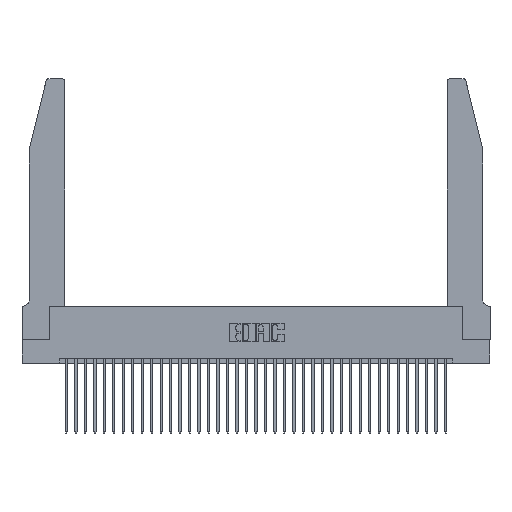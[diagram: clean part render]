
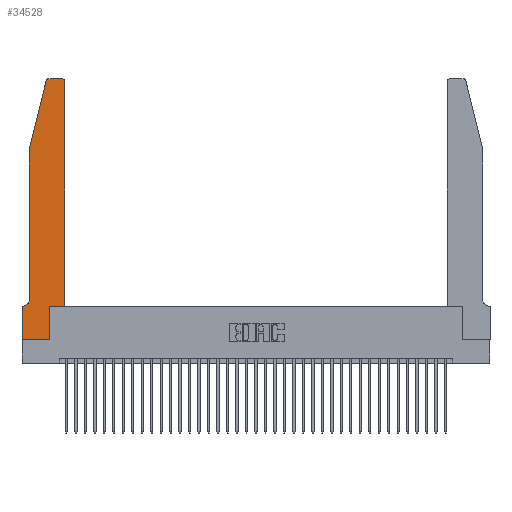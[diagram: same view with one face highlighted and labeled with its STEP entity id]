
A CAD part, top view. The second image highlights one B-rep face of the part: STEP entity #34528.
In plain terms, the highlighted planar face has unit normal (0, 0, 1).
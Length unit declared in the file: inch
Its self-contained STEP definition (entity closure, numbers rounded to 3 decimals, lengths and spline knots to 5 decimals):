
#1128 = VERTEX_POINT ( 'NONE', #4795 ) ;
#1142 = LINE ( 'NONE', #27657, #16571 ) ;
#1581 = CIRCLE ( 'NONE', #6275, 0.03 ) ;
#1779 = VERTEX_POINT ( 'NONE', #21630 ) ;
#1980 = DIRECTION ( 'NONE',  ( 0., 0., 1. ) ) ;
#2965 = EDGE_CURVE ( 'NONE', #1128, #6114, #33499, .T. ) ;
#3066 = DIRECTION ( 'NONE',  ( 0., 1., 0. ) ) ;
#3190 = VECTOR ( 'NONE', #3066, 39.37008 ) ;
#3422 = ORIENTED_EDGE ( 'NONE', *, *, #18337, .T. ) ;
#3525 = VECTOR ( 'NONE', #30238, 39.37008 ) ;
#4795 = CARTESIAN_POINT ( 'NONE',  ( 0., 0., 0.37 ) ) ;
#4916 = CARTESIAN_POINT ( 'NONE',  ( 0., 0.35, 0.37 ) ) ;
#5437 = EDGE_CURVE ( 'NONE', #25850, #1779, #28876, .T. ) ;
#5640 = VERTEX_POINT ( 'NONE', #32951 ) ;
#5647 = ORIENTED_EDGE ( 'NONE', *, *, #13364, .T. ) ;
#5784 = LINE ( 'NONE', #11953, #35310 ) ;
#6114 = VERTEX_POINT ( 'NONE', #34794 ) ;
#6275 = AXIS2_PLACEMENT_3D ( 'NONE', #12377, #32295, #15337 ) ;
#6824 = VERTEX_POINT ( 'NONE', #9285 ) ;
#8579 = CARTESIAN_POINT ( 'NONE',  ( 0.0755, 0.35, 0.37 ) ) ;
#8864 = ORIENTED_EDGE ( 'NONE', *, *, #36455, .T. ) ;
#9285 = CARTESIAN_POINT ( 'NONE',  ( 0.2865, 0.35, 0.37 ) ) ;
#10148 = EDGE_CURVE ( 'NONE', #16829, #36182, #36560, .T. ) ;
#10251 = VERTEX_POINT ( 'NONE', #15287 ) ;
#10747 = PLANE ( 'NONE',  #29472 ) ;
#11078 = CARTESIAN_POINT ( 'NONE',  ( 0.0755, 2., 0.37 ) ) ;
#11239 = LINE ( 'NONE', #24502, #3525 ) ;
#11369 = VECTOR ( 'NONE', #16510, 39.37008 ) ;
#11953 = CARTESIAN_POINT ( 'NONE',  ( 0.4505, 0.35, 0.37 ) ) ;
#12377 = CARTESIAN_POINT ( 'NONE',  ( 0.4205, 2.72, 0.37 ) ) ;
#13364 = EDGE_CURVE ( 'NONE', #36182, #27107, #31470, .T. ) ;
#13442 = CARTESIAN_POINT ( 'NONE',  ( 0.0055, 0.42, 0.37 ) ) ;
#13700 = DIRECTION ( 'NONE',  ( 0., 0., 1. ) ) ;
#14864 = DIRECTION ( 'NONE',  ( 0., -1., 0. ) ) ;
#15026 = DIRECTION ( 'NONE',  ( 1., 0., 0. ) ) ;
#15252 = ORIENTED_EDGE ( 'NONE', *, *, #5437, .T. ) ;
#15287 = CARTESIAN_POINT ( 'NONE',  ( 0.0055, 0.35, 0.37 ) ) ;
#15337 = DIRECTION ( 'NONE',  ( 1., 0., 0. ) ) ;
#16132 = AXIS2_PLACEMENT_3D ( 'NONE', #19301, #1980, #22150 ) ;
#16160 = VECTOR ( 'NONE', #20067, 39.37008 ) ;
#16347 = DIRECTION ( 'NONE',  ( -1., 0., 0. ) ) ;
#16509 = EDGE_CURVE ( 'NONE', #1779, #10251, #27436, .T. ) ;
#16510 = DIRECTION ( 'NONE',  ( -0.239, -0.971, 0. ) ) ;
#16571 = VECTOR ( 'NONE', #33372, 39.37008 ) ;
#16829 = VERTEX_POINT ( 'NONE', #23500 ) ;
#17015 = ORIENTED_EDGE ( 'NONE', *, *, #36226, .T. ) ;
#17113 = FACE_OUTER_BOUND ( 'NONE', #20928, .T. ) ;
#18337 = EDGE_CURVE ( 'NONE', #5640, #1128, #11239, .T. ) ;
#18440 = VECTOR ( 'NONE', #23781, 39.37008 ) ;
#19230 = CARTESIAN_POINT ( 'NONE',  ( 0.0755, 2., 0.37 ) ) ;
#19301 = CARTESIAN_POINT ( 'NONE',  ( 0.284, 2.72, 0.37 ) ) ;
#20067 = DIRECTION ( 'NONE',  ( -1., 0., 0. ) ) ;
#20123 = ORIENTED_EDGE ( 'NONE', *, *, #10148, .T. ) ;
#20928 = EDGE_LOOP ( 'NONE', ( #20123, #5647, #29405, #15252, #30307, #17015, #3422, #33862, #21457, #36520, #8864, #25871 ) ) ;
#21457 = ORIENTED_EDGE ( 'NONE', *, *, #29606, .T. ) ;
#21630 = CARTESIAN_POINT ( 'NONE',  ( 0.0755, 0.42, 0.37 ) ) ;
#22150 = DIRECTION ( 'NONE',  ( 1., 0., 0. ) ) ;
#22224 = VECTOR ( 'NONE', #14864, 39.37008 ) ;
#22645 = CARTESIAN_POINT ( 'NONE',  ( 0.284, 2.75, 0.37 ) ) ;
#23500 = CARTESIAN_POINT ( 'NONE',  ( 0.4205, 2.75, 0.37 ) ) ;
#23781 = DIRECTION ( 'NONE',  ( 1., 0., 0. ) ) ;
#24502 = CARTESIAN_POINT ( 'NONE',  ( 0., 0., 0.37 ) ) ;
#25086 = CARTESIAN_POINT ( 'NONE',  ( 0.4505, 0.35, 0.37 ) ) ;
#25850 = VERTEX_POINT ( 'NONE', #11078 ) ;
#25871 = ORIENTED_EDGE ( 'NONE', *, *, #26482, .T. ) ;
#26066 = CARTESIAN_POINT ( 'NONE',  ( 0.4505, 2.72, 0.37 ) ) ;
#26072 = LINE ( 'NONE', #34483, #3190 ) ;
#26475 = AXIS2_PLACEMENT_3D ( 'NONE', #13442, #33327, #16347 ) ;
#26482 = EDGE_CURVE ( 'NONE', #28957, #16829, #1581, .T. ) ;
#26630 = CARTESIAN_POINT ( 'NONE',  ( 0., 0., 0.37 ) ) ;
#27107 = VERTEX_POINT ( 'NONE', #35474 ) ;
#27436 = CIRCLE ( 'NONE', #26475, 0.07 ) ;
#27657 = CARTESIAN_POINT ( 'NONE',  ( 0.4505, 0.35, 0.37 ) ) ;
#28876 = LINE ( 'NONE', #31840, #22224 ) ;
#28957 = VERTEX_POINT ( 'NONE', #26066 ) ;
#29021 = VECTOR ( 'NONE', #34614, 39.37008 ) ;
#29221 = LINE ( 'NONE', #19230, #11369 ) ;
#29354 = EDGE_CURVE ( 'NONE', #27107, #25850, #29221, .T. ) ;
#29405 = ORIENTED_EDGE ( 'NONE', *, *, #29354, .T. ) ;
#29472 = AXIS2_PLACEMENT_3D ( 'NONE', #4916, #13700, #33556 ) ;
#29606 = EDGE_CURVE ( 'NONE', #6114, #6824, #26072, .T. ) ;
#30238 = DIRECTION ( 'NONE',  ( 0., -1., 0. ) ) ;
#30307 = ORIENTED_EDGE ( 'NONE', *, *, #16509, .T. ) ;
#31242 = LINE ( 'NONE', #8579, #16160 ) ;
#31470 = CIRCLE ( 'NONE', #16132, 0.03 ) ;
#31762 = CARTESIAN_POINT ( 'NONE',  ( 0.2605, 2.75, 0.37 ) ) ;
#31840 = CARTESIAN_POINT ( 'NONE',  ( 0.0755, 2., 0.37 ) ) ;
#32295 = DIRECTION ( 'NONE',  ( 0., 0., 1. ) ) ;
#32951 = CARTESIAN_POINT ( 'NONE',  ( 0., 0.35, 0.37 ) ) ;
#33327 = DIRECTION ( 'NONE',  ( 0., 0., -1. ) ) ;
#33372 = DIRECTION ( 'NONE',  ( 0., 1., 0. ) ) ;
#33499 = LINE ( 'NONE', #26630, #18440 ) ;
#33556 = DIRECTION ( 'NONE',  ( 1., 0., 0. ) ) ;
#33862 = ORIENTED_EDGE ( 'NONE', *, *, #2965, .T. ) ;
#34177 = EDGE_CURVE ( 'NONE', #6824, #36100, #5784, .T. ) ;
#34483 = CARTESIAN_POINT ( 'NONE',  ( 0.2865, 0.35, 0.37 ) ) ;
#34528 = ADVANCED_FACE ( 'NONE', ( #17113 ), #10747, .T. ) ;
#34614 = DIRECTION ( 'NONE',  ( -1., 0., 0. ) ) ;
#34794 = CARTESIAN_POINT ( 'NONE',  ( 0.2865, 0., 0.37 ) ) ;
#35310 = VECTOR ( 'NONE', #15026, 39.37008 ) ;
#35474 = CARTESIAN_POINT ( 'NONE',  ( 0.25487, 2.72718, 0.37 ) ) ;
#36100 = VERTEX_POINT ( 'NONE', #25086 ) ;
#36182 = VERTEX_POINT ( 'NONE', #22645 ) ;
#36226 = EDGE_CURVE ( 'NONE', #10251, #5640, #31242, .T. ) ;
#36455 = EDGE_CURVE ( 'NONE', #36100, #28957, #1142, .T. ) ;
#36520 = ORIENTED_EDGE ( 'NONE', *, *, #34177, .T. ) ;
#36560 = LINE ( 'NONE', #31762, #29021 ) ;
